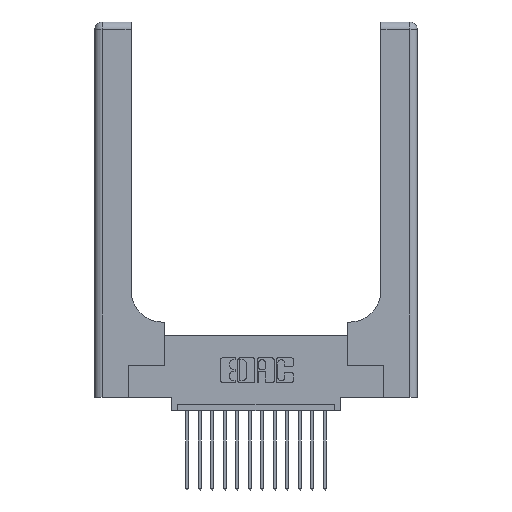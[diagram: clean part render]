
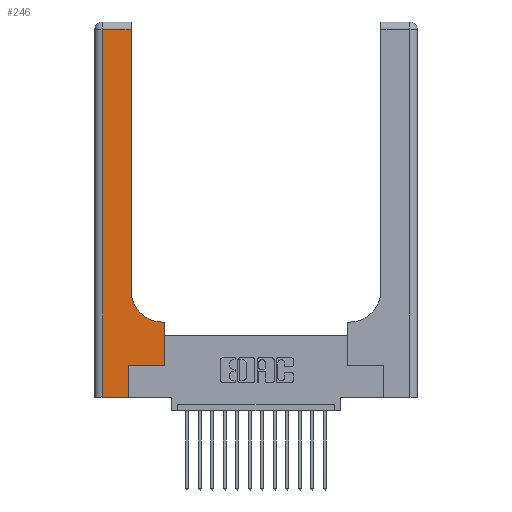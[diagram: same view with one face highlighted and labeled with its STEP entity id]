
A CAD part, top view. The second image highlights one B-rep face of the part: STEP entity #246.
In plain terms, the highlighted planar face has unit normal (0, 0, 1).
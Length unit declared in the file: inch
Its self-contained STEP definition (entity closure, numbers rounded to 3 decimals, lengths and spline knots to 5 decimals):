
#246 = ADVANCED_FACE ( 'NONE', ( #11489 ), #10042, .F. ) ;
#355 = AXIS2_PLACEMENT_3D ( 'NONE', #15663, #15786, #3011 ) ;
#468 = CARTESIAN_POINT ( 'NONE',  ( 0.5585, 0.25, 0.37 ) ) ;
#543 = LINE ( 'NONE', #7575, #13469 ) ;
#580 = CARTESIAN_POINT ( 'NONE',  ( 0., 0., 0.37 ) ) ;
#730 = ORIENTED_EDGE ( 'NONE', *, *, #16799, .T. ) ;
#734 = CARTESIAN_POINT ( 'NONE',  ( 0.5415, 0.6, 0.37 ) ) ;
#1041 = LINE ( 'NONE', #7626, #10159 ) ;
#1345 = CIRCLE ( 'NONE', #8180, 0.25 ) ;
#1597 = ORIENTED_EDGE ( 'NONE', *, *, #12327, .T. ) ;
#1803 = VECTOR ( 'NONE', #18070, 39.37008 ) ;
#2019 = LINE ( 'NONE', #17025, #1803 ) ;
#2474 = LINE ( 'NONE', #7418, #17163 ) ;
#3011 = DIRECTION ( 'NONE',  ( -1., 0., 0. ) ) ;
#3566 = DIRECTION ( 'NONE',  ( -1., 0., 0. ) ) ;
#3737 = ORIENTED_EDGE ( 'NONE', *, *, #14690, .T. ) ;
#4263 = VERTEX_POINT ( 'NONE', #13214 ) ;
#4836 = DIRECTION ( 'NONE',  ( 0., 1., 0. ) ) ;
#6175 = CARTESIAN_POINT ( 'NONE',  ( 0.5585, 0.25, 0.37 ) ) ;
#6191 = EDGE_CURVE ( 'NONE', #6377, #13669, #2474, .T. ) ;
#6377 = VERTEX_POINT ( 'NONE', #8596 ) ;
#6704 = ORIENTED_EDGE ( 'NONE', *, *, #17845, .T. ) ;
#6812 = VERTEX_POINT ( 'NONE', #12723 ) ;
#6959 = CARTESIAN_POINT ( 'NONE',  ( 0.5585, 0.6, 0.37 ) ) ;
#7049 = EDGE_CURVE ( 'NONE', #6812, #7559, #11331, .T. ) ;
#7418 = CARTESIAN_POINT ( 'NONE',  ( 0.269, 0.25, 0.37 ) ) ;
#7553 = VERTEX_POINT ( 'NONE', #734 ) ;
#7559 = VERTEX_POINT ( 'NONE', #10682 ) ;
#7575 = CARTESIAN_POINT ( 'NONE',  ( 0.269, 0., 0.37 ) ) ;
#7626 = CARTESIAN_POINT ( 'NONE',  ( 0., 2.94, 0.37 ) ) ;
#7750 = DIRECTION ( 'NONE',  ( -1., 0., 0. ) ) ;
#8044 = CARTESIAN_POINT ( 'NONE',  ( 0.2915, 2.94, 0.37 ) ) ;
#8051 = DIRECTION ( 'NONE',  ( 0., 0., -1. ) ) ;
#8180 = AXIS2_PLACEMENT_3D ( 'NONE', #15302, #8051, #15235 ) ;
#8334 = EDGE_CURVE ( 'NONE', #18296, #7553, #9753, .T. ) ;
#8596 = CARTESIAN_POINT ( 'NONE',  ( 0.269, 0.25, 0.37 ) ) ;
#8627 = VECTOR ( 'NONE', #3566, 39.37008 ) ;
#9233 = ORIENTED_EDGE ( 'NONE', *, *, #8334, .T. ) ;
#9431 = VECTOR ( 'NONE', #17305, 39.37008 ) ;
#9515 = DIRECTION ( 'NONE',  ( 1., 0., 0. ) ) ;
#9753 = LINE ( 'NONE', #16155, #8627 ) ;
#9790 = EDGE_CURVE ( 'NONE', #4263, #17140, #2019, .T. ) ;
#9795 = EDGE_CURVE ( 'NONE', #7553, #4263, #1345, .T. ) ;
#9891 = LINE ( 'NONE', #10546, #17019 ) ;
#10042 = PLANE ( 'NONE',  #355 ) ;
#10159 = VECTOR ( 'NONE', #7750, 39.37008 ) ;
#10546 = CARTESIAN_POINT ( 'NONE',  ( 0.06, 3., 0.37 ) ) ;
#10608 = DIRECTION ( 'NONE',  ( 0., -1., 0. ) ) ;
#10682 = CARTESIAN_POINT ( 'NONE',  ( 0.269, 0., 0.37 ) ) ;
#10744 = ORIENTED_EDGE ( 'NONE', *, *, #9790, .T. ) ;
#11331 = LINE ( 'NONE', #580, #17793 ) ;
#11489 = FACE_OUTER_BOUND ( 'NONE', #17253, .T. ) ;
#11742 = DIRECTION ( 'NONE',  ( 1., 0., 0. ) ) ;
#12129 = LINE ( 'NONE', #468, #9431 ) ;
#12327 = EDGE_CURVE ( 'NONE', #17140, #14156, #1041, .T. ) ;
#12723 = CARTESIAN_POINT ( 'NONE',  ( 0.06, 0., 0.37 ) ) ;
#13214 = CARTESIAN_POINT ( 'NONE',  ( 0.2915, 0.85, 0.37 ) ) ;
#13469 = VECTOR ( 'NONE', #4836, 39.37008 ) ;
#13669 = VERTEX_POINT ( 'NONE', #6175 ) ;
#14156 = VERTEX_POINT ( 'NONE', #15951 ) ;
#14452 = ORIENTED_EDGE ( 'NONE', *, *, #7049, .T. ) ;
#14690 = EDGE_CURVE ( 'NONE', #13669, #18296, #12129, .T. ) ;
#15235 = DIRECTION ( 'NONE',  ( 1., 0., 0. ) ) ;
#15302 = CARTESIAN_POINT ( 'NONE',  ( 0.5415, 0.85, 0.37 ) ) ;
#15663 = CARTESIAN_POINT ( 'NONE',  ( 0., 3., 0.37 ) ) ;
#15786 = DIRECTION ( 'NONE',  ( 0., 0., -1. ) ) ;
#15951 = CARTESIAN_POINT ( 'NONE',  ( 0.06, 2.94, 0.37 ) ) ;
#16155 = CARTESIAN_POINT ( 'NONE',  ( 0.2915, 0.6, 0.37 ) ) ;
#16799 = EDGE_CURVE ( 'NONE', #14156, #6812, #9891, .T. ) ;
#17019 = VECTOR ( 'NONE', #10608, 39.37008 ) ;
#17025 = CARTESIAN_POINT ( 'NONE',  ( 0.2915, 3., 0.37 ) ) ;
#17140 = VERTEX_POINT ( 'NONE', #8044 ) ;
#17163 = VECTOR ( 'NONE', #11742, 39.37008 ) ;
#17253 = EDGE_LOOP ( 'NONE', ( #10744, #1597, #730, #14452, #6704, #17267, #3737, #9233, #17969 ) ) ;
#17267 = ORIENTED_EDGE ( 'NONE', *, *, #6191, .T. ) ;
#17305 = DIRECTION ( 'NONE',  ( 0., 1., 0. ) ) ;
#17793 = VECTOR ( 'NONE', #9515, 39.37008 ) ;
#17845 = EDGE_CURVE ( 'NONE', #7559, #6377, #543, .T. ) ;
#17969 = ORIENTED_EDGE ( 'NONE', *, *, #9795, .T. ) ;
#18070 = DIRECTION ( 'NONE',  ( 0., 1., 0. ) ) ;
#18296 = VERTEX_POINT ( 'NONE', #6959 ) ;
